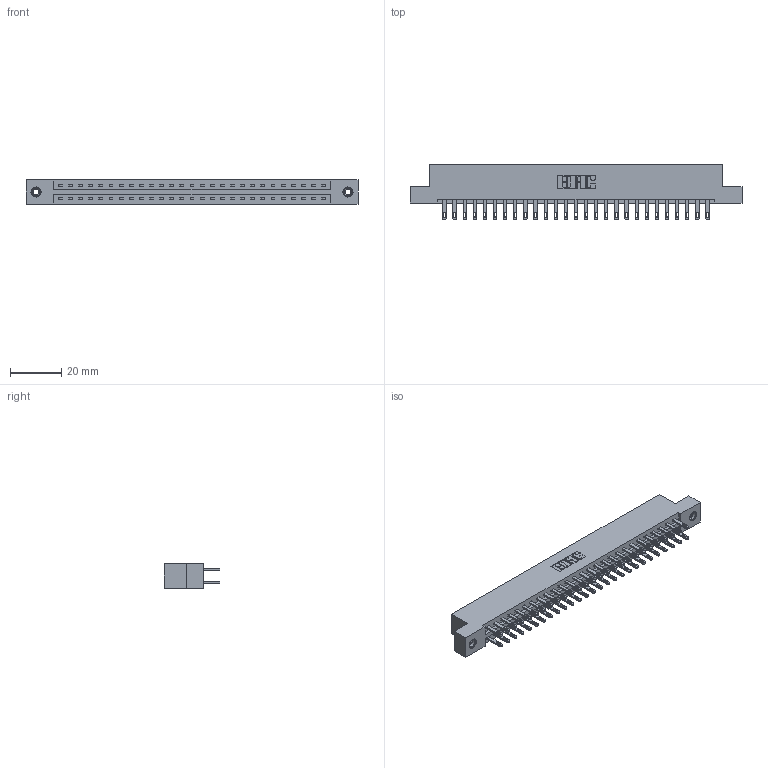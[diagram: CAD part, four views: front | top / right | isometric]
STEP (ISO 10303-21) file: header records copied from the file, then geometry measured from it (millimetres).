
FILE_DESCRIPTION (( 'STEP AP203' ), '1' );
FILE_NAME ('337-054-500-208.STEP', '2019-10-09T17:33:11', ( '' ), ( '' ), 'SwSTEP 2.0', 'SolidWorks 2016', '' );
FILE_SCHEMA (( 'CONFIG_CONTROL_DESIGN' ));
Length unit declared in the file: inch
Products named in the file (4): 337-054-500-208; 345-250-001_345-250-003-102; 337 Part_Flush Mounting Lugs - 0.156 Dia-TI; 345-292-001_345-293-100
Assembly tree (57 placements, depth 2):
  337-054-500-208
    337 Part_Flush Mounting Lugs - 0.156 Dia-TI
    345-292-001_345-293-100  x54
    345-250-001_345-250-003-102  x2
Bounding box: 130 x 21.85 x 9.4 mm (x, y, z)
Volume: 13659 mm3; surface area: 15918.9 mm2
Topology: 57 solids, 57 shells, 2874 faces, 8709 edges, 5798 vertices
Faces by surface type: plane 1830, cylinder 1028, cone 12, torus 4
Entity records: 23990 total; most frequent: CARTESIAN_POINT 4033, ORIENTED_EDGE 3962, DIRECTION 3491, EDGE_CURVE 1981, VECTOR 1829, LINE 1829, VERTEX_POINT 1316, AXIS2_PLACEMENT_3D 831
